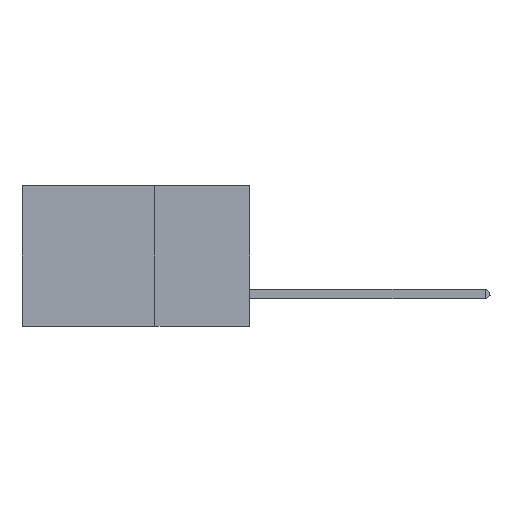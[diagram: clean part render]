
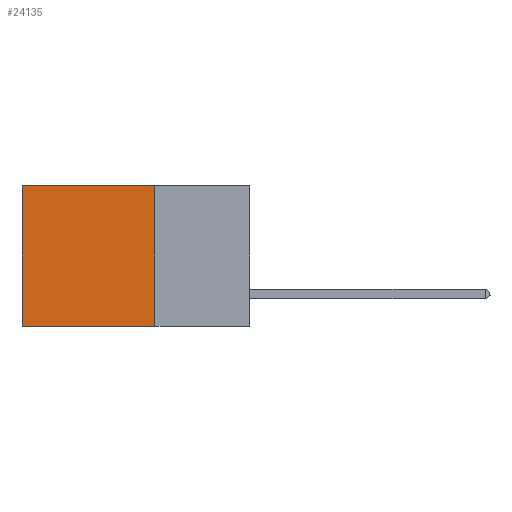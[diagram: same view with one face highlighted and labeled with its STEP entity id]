
A CAD part, left-side view. The second image highlights one B-rep face of the part: STEP entity #24135.
In plain terms, the highlighted planar face has unit normal (-1, 0, 0).
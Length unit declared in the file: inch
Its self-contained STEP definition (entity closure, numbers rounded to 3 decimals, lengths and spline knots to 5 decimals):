
#2220 = DIRECTION ( 'NONE',  ( 0., 1., 0. ) ) ;
#2914 = EDGE_CURVE ( 'NONE', #7013, #8639, #27760, .T. ) ;
#3316 = DIRECTION ( 'NONE',  ( 1., 0., 0. ) ) ;
#4087 = PLANE ( 'NONE',  #7348 ) ;
#4098 = DIRECTION ( 'NONE',  ( 0., 1., 0. ) ) ;
#4182 = VECTOR ( 'NONE', #2220, 39.37008 ) ;
#5260 = EDGE_CURVE ( 'NONE', #8458, #8639, #18866, .T. ) ;
#7013 = VERTEX_POINT ( 'NONE', #12003 ) ;
#7348 = AXIS2_PLACEMENT_3D ( 'NONE', #26577, #3316, #24403 ) ;
#7741 = CARTESIAN_POINT ( 'NONE',  ( 0.2875, 0.25, 0. ) ) ;
#8458 = VERTEX_POINT ( 'NONE', #8845 ) ;
#8639 = VERTEX_POINT ( 'NONE', #22421 ) ;
#8845 = CARTESIAN_POINT ( 'NONE',  ( 0.2875, 0.6, 0. ) ) ;
#10020 = ORIENTED_EDGE ( 'NONE', *, *, #28008, .T. ) ;
#11073 = VERTEX_POINT ( 'NONE', #7741 ) ;
#12003 = CARTESIAN_POINT ( 'NONE',  ( 0.2875, 0.25, -0.37 ) ) ;
#13628 = VECTOR ( 'NONE', #20448, 39.37008 ) ;
#17606 = ORIENTED_EDGE ( 'NONE', *, *, #28135, .F. ) ;
#18469 = CARTESIAN_POINT ( 'NONE',  ( 0.2875, 0.6, 0. ) ) ;
#18618 = VECTOR ( 'NONE', #4098, 39.37008 ) ;
#18866 = LINE ( 'NONE', #18469, #25911 ) ;
#19837 = ORIENTED_EDGE ( 'NONE', *, *, #2914, .F. ) ;
#20448 = DIRECTION ( 'NONE',  ( 0., 0., -1. ) ) ;
#20819 = CARTESIAN_POINT ( 'NONE',  ( 0.2875, 0.25, 0. ) ) ;
#21737 = CARTESIAN_POINT ( 'NONE',  ( 0.2875, 0.25, -0.37 ) ) ;
#22421 = CARTESIAN_POINT ( 'NONE',  ( 0.2875, 0.6, -0.37 ) ) ;
#23151 = DIRECTION ( 'NONE',  ( 0., 0., -1. ) ) ;
#24135 = ADVANCED_FACE ( 'NONE', ( #28696 ), #4087, .F. ) ;
#24170 = LINE ( 'NONE', #20819, #4182 ) ;
#24403 = DIRECTION ( 'NONE',  ( 0., 0., -1. ) ) ;
#25620 = LINE ( 'NONE', #27075, #13628 ) ;
#25911 = VECTOR ( 'NONE', #23151, 39.37008 ) ;
#26577 = CARTESIAN_POINT ( 'NONE',  ( 0.2875, 0.25, 0. ) ) ;
#27075 = CARTESIAN_POINT ( 'NONE',  ( 0.2875, 0.25, 0. ) ) ;
#27760 = LINE ( 'NONE', #21737, #18618 ) ;
#28008 = EDGE_CURVE ( 'NONE', #11073, #8458, #24170, .T. ) ;
#28135 = EDGE_CURVE ( 'NONE', #11073, #7013, #25620, .T. ) ;
#28585 = EDGE_LOOP ( 'NONE', ( #28866, #19837, #17606, #10020 ) ) ;
#28696 = FACE_OUTER_BOUND ( 'NONE', #28585, .T. ) ;
#28866 = ORIENTED_EDGE ( 'NONE', *, *, #5260, .T. ) ;
